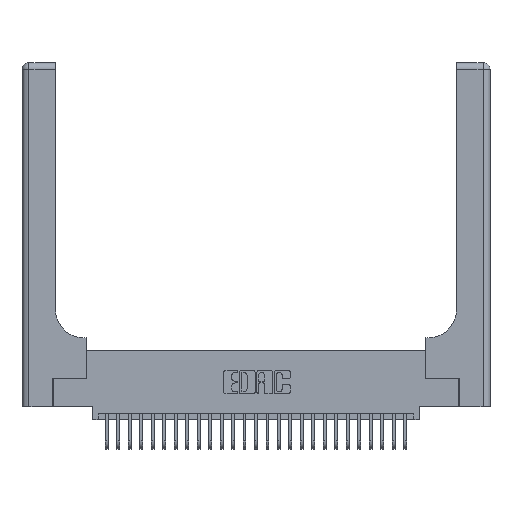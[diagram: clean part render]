
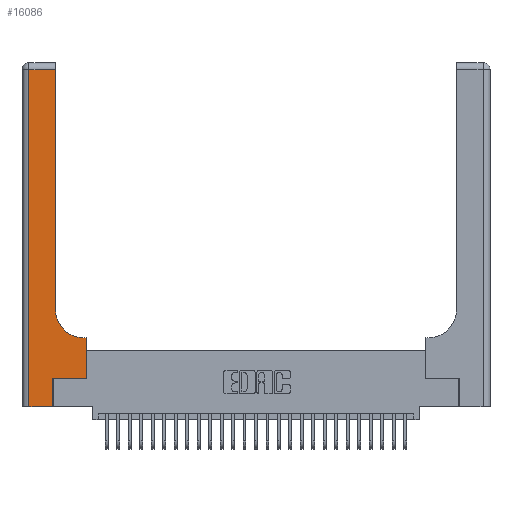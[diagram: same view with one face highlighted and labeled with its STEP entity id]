
A CAD part, top view. The second image highlights one B-rep face of the part: STEP entity #16086.
In plain terms, the highlighted planar face has unit normal (0, 0, 1).
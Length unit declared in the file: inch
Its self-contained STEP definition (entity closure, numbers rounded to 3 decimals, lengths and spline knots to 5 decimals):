
#1001 = CARTESIAN_POINT ( 'NONE',  ( 0.5415, 0.85, 0.37 ) ) ;
#1162 = EDGE_LOOP ( 'NONE', ( #14940, #24085, #13957, #25089, #18755, #25456, #11102, #5334, #11904 ) ) ;
#1226 = VERTEX_POINT ( 'NONE', #11329 ) ;
#1448 = AXIS2_PLACEMENT_3D ( 'NONE', #1001, #15938, #3159 ) ;
#1601 = EDGE_CURVE ( 'NONE', #20171, #18024, #4842, .T. ) ;
#1891 = VECTOR ( 'NONE', #24728, 39.37008 ) ;
#2186 = VERTEX_POINT ( 'NONE', #23758 ) ;
#2936 = EDGE_CURVE ( 'NONE', #8226, #2186, #5429, .T. ) ;
#3159 = DIRECTION ( 'NONE',  ( 1., 0., 0. ) ) ;
#3232 = CARTESIAN_POINT ( 'NONE',  ( 0.06, 0., 0.37 ) ) ;
#3728 = CARTESIAN_POINT ( 'NONE',  ( 0.06, 2.94, 0.37 ) ) ;
#4540 = EDGE_CURVE ( 'NONE', #10535, #10959, #11073, .T. ) ;
#4569 = PLANE ( 'NONE',  #24421 ) ;
#4642 = DIRECTION ( 'NONE',  ( 0., 1., 0. ) ) ;
#4653 = CARTESIAN_POINT ( 'NONE',  ( 0., 3., 0.37 ) ) ;
#4776 = LINE ( 'NONE', #17279, #21251 ) ;
#4842 = LINE ( 'NONE', #8303, #26302 ) ;
#5334 = ORIENTED_EDGE ( 'NONE', *, *, #22356, .T. ) ;
#5429 = LINE ( 'NONE', #24098, #10445 ) ;
#6681 = CARTESIAN_POINT ( 'NONE',  ( 0.269, 0.25, 0.37 ) ) ;
#6790 = DIRECTION ( 'NONE',  ( 0., 0., -1. ) ) ;
#8094 = FACE_OUTER_BOUND ( 'NONE', #1162, .T. ) ;
#8226 = VERTEX_POINT ( 'NONE', #13913 ) ;
#8303 = CARTESIAN_POINT ( 'NONE',  ( 0.2915, 3., 0.37 ) ) ;
#10445 = VECTOR ( 'NONE', #19888, 39.37008 ) ;
#10463 = DIRECTION ( 'NONE',  ( 0., 1., 0. ) ) ;
#10507 = VECTOR ( 'NONE', #19168, 39.37008 ) ;
#10535 = VERTEX_POINT ( 'NONE', #3728 ) ;
#10959 = VERTEX_POINT ( 'NONE', #3232 ) ;
#11073 = LINE ( 'NONE', #19334, #21852 ) ;
#11102 = ORIENTED_EDGE ( 'NONE', *, *, #2936, .T. ) ;
#11329 = CARTESIAN_POINT ( 'NONE',  ( 0.5415, 0.6, 0.37 ) ) ;
#11685 = DIRECTION ( 'NONE',  ( -1., 0., 0. ) ) ;
#11748 = CARTESIAN_POINT ( 'NONE',  ( 0.2915, 2.94, 0.37 ) ) ;
#11904 = ORIENTED_EDGE ( 'NONE', *, *, #18536, .T. ) ;
#12434 = VECTOR ( 'NONE', #19832, 39.37008 ) ;
#12921 = DIRECTION ( 'NONE',  ( 0., -1., 0. ) ) ;
#13094 = LINE ( 'NONE', #17646, #12434 ) ;
#13178 = VERTEX_POINT ( 'NONE', #17003 ) ;
#13700 = LINE ( 'NONE', #13816, #20150 ) ;
#13816 = CARTESIAN_POINT ( 'NONE',  ( 0., 2.94, 0.37 ) ) ;
#13913 = CARTESIAN_POINT ( 'NONE',  ( 0.5585, 0.25, 0.37 ) ) ;
#13957 = ORIENTED_EDGE ( 'NONE', *, *, #4540, .T. ) ;
#14940 = ORIENTED_EDGE ( 'NONE', *, *, #1601, .T. ) ;
#15090 = EDGE_CURVE ( 'NONE', #13178, #25514, #4776, .T. ) ;
#15938 = DIRECTION ( 'NONE',  ( 0., 0., -1. ) ) ;
#16086 = ADVANCED_FACE ( 'NONE', ( #8094 ), #4569, .F. ) ;
#16610 = EDGE_CURVE ( 'NONE', #25514, #8226, #13094, .T. ) ;
#16970 = CARTESIAN_POINT ( 'NONE',  ( 0.2915, 0.6, 0.37 ) ) ;
#17003 = CARTESIAN_POINT ( 'NONE',  ( 0.269, 0., 0.37 ) ) ;
#17279 = CARTESIAN_POINT ( 'NONE',  ( 0.269, 0., 0.37 ) ) ;
#17443 = EDGE_CURVE ( 'NONE', #18024, #10535, #13700, .T. ) ;
#17646 = CARTESIAN_POINT ( 'NONE',  ( 0.269, 0.25, 0.37 ) ) ;
#18024 = VERTEX_POINT ( 'NONE', #11748 ) ;
#18536 = EDGE_CURVE ( 'NONE', #1226, #20171, #22430, .T. ) ;
#18755 = ORIENTED_EDGE ( 'NONE', *, *, #15090, .T. ) ;
#19168 = DIRECTION ( 'NONE',  ( -1., 0., 0. ) ) ;
#19334 = CARTESIAN_POINT ( 'NONE',  ( 0.06, 3., 0.37 ) ) ;
#19832 = DIRECTION ( 'NONE',  ( 1., 0., 0. ) ) ;
#19888 = DIRECTION ( 'NONE',  ( 0., 1., 0. ) ) ;
#20150 = VECTOR ( 'NONE', #11685, 39.37008 ) ;
#20171 = VERTEX_POINT ( 'NONE', #21923 ) ;
#21251 = VECTOR ( 'NONE', #4642, 39.37008 ) ;
#21831 = DIRECTION ( 'NONE',  ( -1., 0., 0. ) ) ;
#21852 = VECTOR ( 'NONE', #12921, 39.37008 ) ;
#21923 = CARTESIAN_POINT ( 'NONE',  ( 0.2915, 0.85, 0.37 ) ) ;
#21948 = LINE ( 'NONE', #16970, #10507 ) ;
#22356 = EDGE_CURVE ( 'NONE', #2186, #1226, #21948, .T. ) ;
#22430 = CIRCLE ( 'NONE', #1448, 0.25 ) ;
#22577 = CARTESIAN_POINT ( 'NONE',  ( 0., 0., 0.37 ) ) ;
#23365 = LINE ( 'NONE', #22577, #1891 ) ;
#23758 = CARTESIAN_POINT ( 'NONE',  ( 0.5585, 0.6, 0.37 ) ) ;
#24085 = ORIENTED_EDGE ( 'NONE', *, *, #17443, .T. ) ;
#24098 = CARTESIAN_POINT ( 'NONE',  ( 0.5585, 0.25, 0.37 ) ) ;
#24421 = AXIS2_PLACEMENT_3D ( 'NONE', #4653, #6790, #21831 ) ;
#24728 = DIRECTION ( 'NONE',  ( 1., 0., 0. ) ) ;
#25089 = ORIENTED_EDGE ( 'NONE', *, *, #27729, .T. ) ;
#25456 = ORIENTED_EDGE ( 'NONE', *, *, #16610, .T. ) ;
#25514 = VERTEX_POINT ( 'NONE', #6681 ) ;
#26302 = VECTOR ( 'NONE', #10463, 39.37008 ) ;
#27729 = EDGE_CURVE ( 'NONE', #10959, #13178, #23365, .T. ) ;
